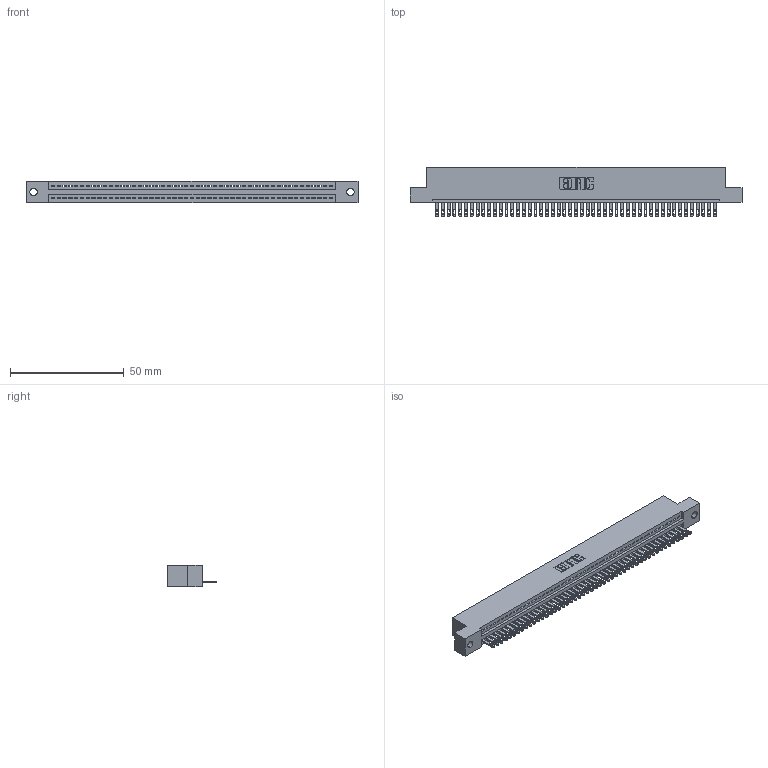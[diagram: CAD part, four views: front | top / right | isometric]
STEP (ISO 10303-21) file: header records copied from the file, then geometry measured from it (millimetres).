
FILE_DESCRIPTION (( 'STEP AP203' ), '1' );
FILE_NAME ('345-049-500-102.STEP', '2018-09-12T12:15:50', ( '' ), ( '' ), 'SwSTEP 2.0', 'SolidWorks 2016', '' );
FILE_SCHEMA (( 'CONFIG_CONTROL_DESIGN' ));
Length unit declared in the file: inch
Products named in the file (3): 345 Part_Flush Mounting Lugs - 0.128 Dia; 345-292-001_345-293-100; 345-049-500-102
Assembly tree (50 placements, depth 2):
  345-049-500-102
    345 Part_Flush Mounting Lugs - 0.128 Dia
    345-292-001_345-293-100  x49
Bounding box: 145.67 x 21.51 x 9.4 mm (x, y, z)
Volume: 13886.8 mm3; surface area: 18387.9 mm2
Topology: 50 solids, 50 shells, 2772 faces, 8573 edges, 5714 vertices
Faces by surface type: plane 1746, cylinder 1026
Entity records: 35869 total; most frequent: CARTESIAN_POINT 6219, ORIENTED_EDGE 6202, DIRECTION 5423, EDGE_CURVE 3101, VECTOR 2769, LINE 2769, VERTEX_POINT 2066, AXIS2_PLACEMENT_3D 1327
